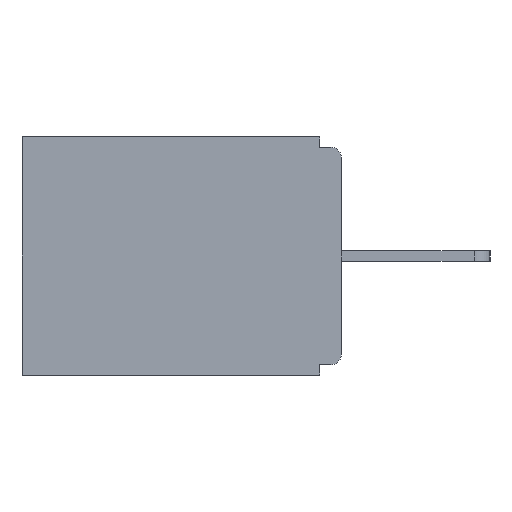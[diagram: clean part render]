
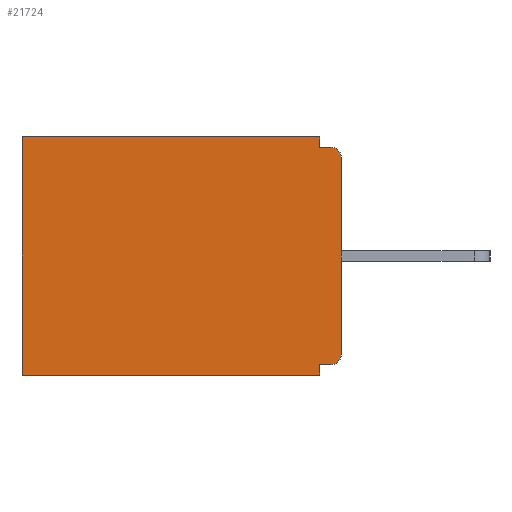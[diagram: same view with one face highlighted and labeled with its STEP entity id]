
A CAD part, left-side view. The second image highlights one B-rep face of the part: STEP entity #21724.
In plain terms, the highlighted planar face has unit normal (-1, 0, 0).
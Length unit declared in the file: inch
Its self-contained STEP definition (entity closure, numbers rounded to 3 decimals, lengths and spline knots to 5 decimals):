
#465 = VERTEX_POINT ( 'NONE', #15547 ) ;
#1514 = DIRECTION ( 'NONE',  ( 0., 0., -1. ) ) ;
#1922 = DIRECTION ( 'NONE',  ( 0., 1., 0. ) ) ;
#2066 = CARTESIAN_POINT ( 'NONE',  ( 0.298, 0., -0.343 ) ) ;
#2305 = VECTOR ( 'NONE', #4699, 39.37008 ) ;
#2354 = CIRCLE ( 'NONE', #6696, 0.015 ) ;
#2378 = LINE ( 'NONE', #4370, #8520 ) ;
#2430 = LINE ( 'NONE', #4545, #6921 ) ;
#2452 = VERTEX_POINT ( 'NONE', #21059 ) ;
#2909 = EDGE_CURVE ( 'NONE', #12161, #5018, #2378, .T. ) ;
#3001 = AXIS2_PLACEMENT_3D ( 'NONE', #19946, #8589, #8706 ) ;
#3428 = DIRECTION ( 'NONE',  ( -1., 0., 0. ) ) ;
#3780 = DIRECTION ( 'NONE',  ( 0., 0., -1. ) ) ;
#4370 = CARTESIAN_POINT ( 'NONE',  ( 0.298, 0., -0.328 ) ) ;
#4544 = VERTEX_POINT ( 'NONE', #20409 ) ;
#4545 = CARTESIAN_POINT ( 'NONE',  ( 0.298, 0.46, 0. ) ) ;
#4699 = DIRECTION ( 'NONE',  ( 0., 0., -1. ) ) ;
#4828 = VERTEX_POINT ( 'NONE', #14906 ) ;
#4885 = PLANE ( 'NONE',  #3001 ) ;
#4913 = DIRECTION ( 'NONE',  ( 0., 0., -1. ) ) ;
#5018 = VERTEX_POINT ( 'NONE', #16229 ) ;
#5114 = CARTESIAN_POINT ( 'NONE',  ( 0.298, 0.031, 0. ) ) ;
#5353 = LINE ( 'NONE', #20425, #16924 ) ;
#5700 = EDGE_CURVE ( 'NONE', #7552, #11880, #18834, .T. ) ;
#6504 = EDGE_CURVE ( 'NONE', #465, #12649, #9371, .T. ) ;
#6575 = EDGE_CURVE ( 'NONE', #11880, #12649, #2430, .T. ) ;
#6691 = DIRECTION ( 'NONE',  ( 0., 0., -1. ) ) ;
#6696 = AXIS2_PLACEMENT_3D ( 'NONE', #22315, #3428, #4913 ) ;
#6921 = VECTOR ( 'NONE', #8237, 39.37008 ) ;
#6999 = VECTOR ( 'NONE', #3780, 39.37008 ) ;
#7173 = VECTOR ( 'NONE', #1514, 39.37008 ) ;
#7552 = VERTEX_POINT ( 'NONE', #5114 ) ;
#7911 = EDGE_CURVE ( 'NONE', #12161, #4544, #16406, .T. ) ;
#8237 = DIRECTION ( 'NONE',  ( 0., 0., -1. ) ) ;
#8252 = CARTESIAN_POINT ( 'NONE',  ( 0.298, 0.46, -0.343 ) ) ;
#8520 = VECTOR ( 'NONE', #18938, 39.37008 ) ;
#8589 = DIRECTION ( 'NONE',  ( 1., 0., 0. ) ) ;
#8673 = VECTOR ( 'NONE', #1922, 39.37008 ) ;
#8706 = DIRECTION ( 'NONE',  ( 0., 0., -1. ) ) ;
#8940 = CARTESIAN_POINT ( 'NONE',  ( 0.298, 0.46, 0. ) ) ;
#9043 = EDGE_CURVE ( 'NONE', #4828, #4544, #20698, .T. ) ;
#9285 = VERTEX_POINT ( 'NONE', #23286 ) ;
#9366 = EDGE_LOOP ( 'NONE', ( #14120, #22734, #16552, #21502, #23037, #17541, #12819, #13361, #11435, #17787 ) ) ;
#9371 = LINE ( 'NONE', #2066, #20199 ) ;
#10676 = EDGE_CURVE ( 'NONE', #7552, #2452, #11976, .T. ) ;
#10751 = LINE ( 'NONE', #23839, #7173 ) ;
#11103 = EDGE_CURVE ( 'NONE', #2452, #9285, #5353, .T. ) ;
#11418 = EDGE_CURVE ( 'NONE', #4828, #9285, #2354, .T. ) ;
#11435 = ORIENTED_EDGE ( 'NONE', *, *, #7911, .T. ) ;
#11880 = VERTEX_POINT ( 'NONE', #8940 ) ;
#11976 = LINE ( 'NONE', #19496, #2305 ) ;
#12161 = VERTEX_POINT ( 'NONE', #16047 ) ;
#12484 = CARTESIAN_POINT ( 'NONE',  ( 0.298, 0.015, -0.313 ) ) ;
#12649 = VERTEX_POINT ( 'NONE', #8252 ) ;
#12819 = ORIENTED_EDGE ( 'NONE', *, *, #13909, .F. ) ;
#13281 = CARTESIAN_POINT ( 'NONE',  ( 0.298, 0., 0. ) ) ;
#13361 = ORIENTED_EDGE ( 'NONE', *, *, #2909, .F. ) ;
#13635 = AXIS2_PLACEMENT_3D ( 'NONE', #12484, #13974, #6691 ) ;
#13909 = EDGE_CURVE ( 'NONE', #5018, #465, #10751, .T. ) ;
#13974 = DIRECTION ( 'NONE',  ( -1., 0., 0. ) ) ;
#14120 = ORIENTED_EDGE ( 'NONE', *, *, #11418, .T. ) ;
#14142 = FACE_OUTER_BOUND ( 'NONE', #9366, .T. ) ;
#14906 = CARTESIAN_POINT ( 'NONE',  ( 0.298, 0., -0.03 ) ) ;
#15153 = DIRECTION ( 'NONE',  ( 0., 1., 0. ) ) ;
#15547 = CARTESIAN_POINT ( 'NONE',  ( 0.298, 0.031, -0.343 ) ) ;
#16047 = CARTESIAN_POINT ( 'NONE',  ( 0.298, 0.015, -0.328 ) ) ;
#16229 = CARTESIAN_POINT ( 'NONE',  ( 0.298, 0.031, -0.328 ) ) ;
#16406 = CIRCLE ( 'NONE', #13635, 0.015 ) ;
#16552 = ORIENTED_EDGE ( 'NONE', *, *, #10676, .F. ) ;
#16575 = DIRECTION ( 'NONE',  ( 0., -1., 0. ) ) ;
#16924 = VECTOR ( 'NONE', #16575, 39.37008 ) ;
#17541 = ORIENTED_EDGE ( 'NONE', *, *, #6504, .F. ) ;
#17787 = ORIENTED_EDGE ( 'NONE', *, *, #9043, .F. ) ;
#18834 = LINE ( 'NONE', #13281, #8673 ) ;
#18938 = DIRECTION ( 'NONE',  ( 0., 1., 0. ) ) ;
#19496 = CARTESIAN_POINT ( 'NONE',  ( 0.298, 0.031, -0.343 ) ) ;
#19946 = CARTESIAN_POINT ( 'NONE',  ( 0.298, 0., 0. ) ) ;
#20199 = VECTOR ( 'NONE', #15153, 39.37008 ) ;
#20409 = CARTESIAN_POINT ( 'NONE',  ( 0.298, 0., -0.313 ) ) ;
#20425 = CARTESIAN_POINT ( 'NONE',  ( 0.298, 0., -0.015 ) ) ;
#20698 = LINE ( 'NONE', #20832, #6999 ) ;
#20832 = CARTESIAN_POINT ( 'NONE',  ( 0.298, 0., 0. ) ) ;
#21059 = CARTESIAN_POINT ( 'NONE',  ( 0.298, 0.031, -0.015 ) ) ;
#21502 = ORIENTED_EDGE ( 'NONE', *, *, #5700, .T. ) ;
#21724 = ADVANCED_FACE ( 'NONE', ( #14142 ), #4885, .F. ) ;
#22315 = CARTESIAN_POINT ( 'NONE',  ( 0.298, 0.015, -0.03 ) ) ;
#22734 = ORIENTED_EDGE ( 'NONE', *, *, #11103, .F. ) ;
#23037 = ORIENTED_EDGE ( 'NONE', *, *, #6575, .T. ) ;
#23286 = CARTESIAN_POINT ( 'NONE',  ( 0.298, 0.015, -0.015 ) ) ;
#23839 = CARTESIAN_POINT ( 'NONE',  ( 0.298, 0.031, -0.343 ) ) ;
